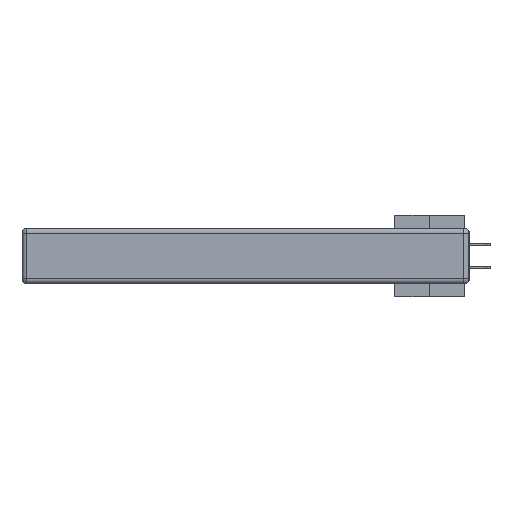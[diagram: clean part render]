
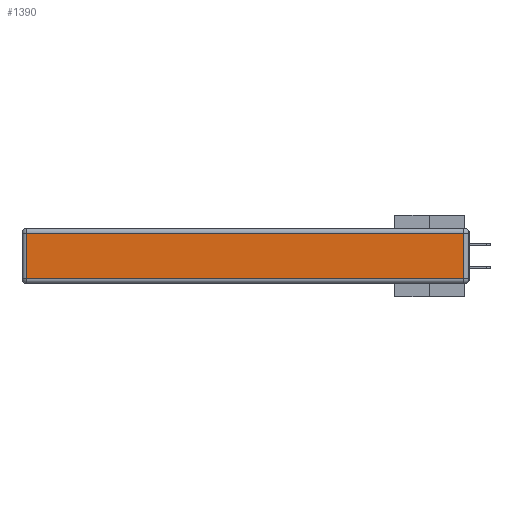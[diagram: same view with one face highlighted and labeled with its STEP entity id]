
A CAD part, left-side view. The second image highlights one B-rep face of the part: STEP entity #1390.
In plain terms, the highlighted planar face has unit normal (-1, 0, 0).
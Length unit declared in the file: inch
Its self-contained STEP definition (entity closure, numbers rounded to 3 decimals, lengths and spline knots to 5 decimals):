
#1390 = ADVANCED_FACE ( 'NONE', ( #35058 ), #42753, .T. ) ;
#2667 = EDGE_LOOP ( 'NONE', ( #38520, #22260, #41402, #5303 ) ) ;
#4216 = CARTESIAN_POINT ( 'NONE',  ( 0., 0.03, -0.343 ) ) ;
#5303 = ORIENTED_EDGE ( 'NONE', *, *, #7081, .T. ) ;
#5735 = DIRECTION ( 'NONE',  ( 0., 0., -1. ) ) ;
#7081 = EDGE_CURVE ( 'NONE', #12799, #20446, #29184, .T. ) ;
#8338 = VECTOR ( 'NONE', #5735, 39.37008 ) ;
#8966 = LINE ( 'NONE', #4216, #46089 ) ;
#10361 = CARTESIAN_POINT ( 'NONE',  ( 0., 0.03, -0.313 ) ) ;
#10395 = CARTESIAN_POINT ( 'NONE',  ( 0., 0., -0.313 ) ) ;
#12799 = VERTEX_POINT ( 'NONE', #21861 ) ;
#13429 = CARTESIAN_POINT ( 'NONE',  ( 0., 0., -0.343 ) ) ;
#17465 = DIRECTION ( 'NONE',  ( -1., 0., 0. ) ) ;
#20446 = VERTEX_POINT ( 'NONE', #34888 ) ;
#21777 = DIRECTION ( 'NONE',  ( 0., 1., 0. ) ) ;
#21861 = CARTESIAN_POINT ( 'NONE',  ( 0., 2.72, -0.03 ) ) ;
#22260 = ORIENTED_EDGE ( 'NONE', *, *, #22489, .T. ) ;
#22411 = EDGE_CURVE ( 'NONE', #32712, #12799, #47881, .T. ) ;
#22489 = EDGE_CURVE ( 'NONE', #41795, #32712, #8966, .T. ) ;
#27780 = CARTESIAN_POINT ( 'NONE',  ( 0., 2.72, -0.343 ) ) ;
#28577 = EDGE_CURVE ( 'NONE', #20446, #41795, #41545, .T. ) ;
#29102 = DIRECTION ( 'NONE',  ( 0., -1., 0. ) ) ;
#29184 = LINE ( 'NONE', #27780, #8338 ) ;
#29512 = AXIS2_PLACEMENT_3D ( 'NONE', #13429, #17465, #43401 ) ;
#32712 = VERTEX_POINT ( 'NONE', #37402 ) ;
#34888 = CARTESIAN_POINT ( 'NONE',  ( 0., 2.72, -0.313 ) ) ;
#35058 = FACE_OUTER_BOUND ( 'NONE', #2667, .T. ) ;
#37402 = CARTESIAN_POINT ( 'NONE',  ( 0., 0.03, -0.03 ) ) ;
#37473 = VECTOR ( 'NONE', #29102, 39.37008 ) ;
#37948 = VECTOR ( 'NONE', #21777, 39.37008 ) ;
#38520 = ORIENTED_EDGE ( 'NONE', *, *, #28577, .T. ) ;
#41067 = DIRECTION ( 'NONE',  ( 0., 0., 1. ) ) ;
#41402 = ORIENTED_EDGE ( 'NONE', *, *, #22411, .T. ) ;
#41545 = LINE ( 'NONE', #10395, #37473 ) ;
#41795 = VERTEX_POINT ( 'NONE', #10361 ) ;
#42753 = PLANE ( 'NONE',  #29512 ) ;
#43401 = DIRECTION ( 'NONE',  ( 0., 0., 1. ) ) ;
#44005 = CARTESIAN_POINT ( 'NONE',  ( 0., 2.75, -0.03 ) ) ;
#46089 = VECTOR ( 'NONE', #41067, 39.37008 ) ;
#47881 = LINE ( 'NONE', #44005, #37948 ) ;
